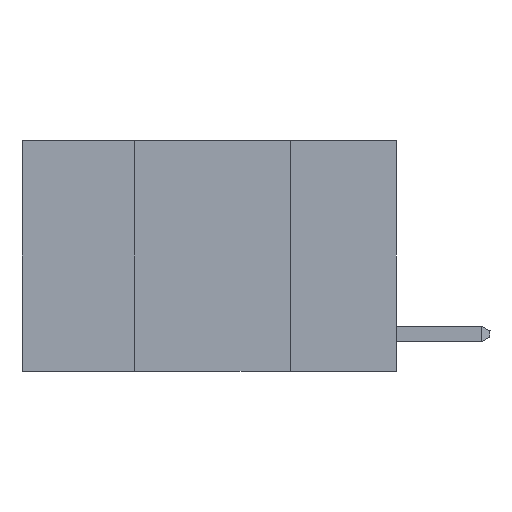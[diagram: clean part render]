
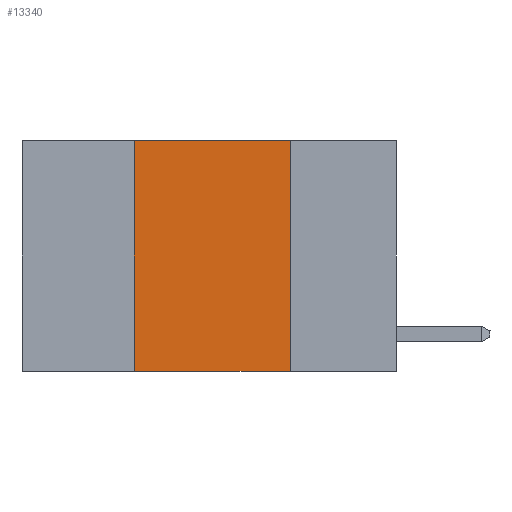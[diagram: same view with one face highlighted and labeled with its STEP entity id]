
A CAD part, left-side view. The second image highlights one B-rep face of the part: STEP entity #13340.
In plain terms, the highlighted planar face has unit normal (-1, 0, 0).
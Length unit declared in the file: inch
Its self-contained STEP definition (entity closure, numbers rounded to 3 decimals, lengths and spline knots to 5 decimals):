
#36 = DIRECTION ( 'NONE',  ( 0., -1., 0. ) ) ;
#970 = EDGE_CURVE ( 'NONE', #9178, #13717, #9839, .T. ) ;
#1294 = VERTEX_POINT ( 'NONE', #14697 ) ;
#2353 = ORIENTED_EDGE ( 'NONE', *, *, #5533, .F. ) ;
#3614 = VECTOR ( 'NONE', #36, 39.37008 ) ;
#3980 = VECTOR ( 'NONE', #14433, 39.37008 ) ;
#4846 = AXIS2_PLACEMENT_3D ( 'NONE', #16590, #19564, #6936 ) ;
#5307 = PLANE ( 'NONE',  #4846 ) ;
#5533 = EDGE_CURVE ( 'NONE', #12806, #9178, #7271, .T. ) ;
#6019 = ORIENTED_EDGE ( 'NONE', *, *, #19326, .F. ) ;
#6936 = DIRECTION ( 'NONE',  ( 0., 0., -1. ) ) ;
#7180 = CARTESIAN_POINT ( 'NONE',  ( 0., 0.6, 0. ) ) ;
#7271 = LINE ( 'NONE', #19435, #3980 ) ;
#8735 = FACE_OUTER_BOUND ( 'NONE', #16406, .T. ) ;
#8837 = DIRECTION ( 'NONE',  ( 0., -1., 0. ) ) ;
#9178 = VERTEX_POINT ( 'NONE', #11370 ) ;
#9364 = CARTESIAN_POINT ( 'NONE',  ( 0., 0.6, -0.37 ) ) ;
#9707 = VECTOR ( 'NONE', #18661, 39.37008 ) ;
#9781 = CARTESIAN_POINT ( 'NONE',  ( 0., 0.17, 0. ) ) ;
#9839 = LINE ( 'NONE', #7180, #17829 ) ;
#9998 = CARTESIAN_POINT ( 'NONE',  ( 0., 0.17, 0. ) ) ;
#11370 = CARTESIAN_POINT ( 'NONE',  ( 0., 0.42, 0. ) ) ;
#12806 = VERTEX_POINT ( 'NONE', #15641 ) ;
#13340 = ADVANCED_FACE ( 'NONE', ( #8735 ), #5307, .F. ) ;
#13495 = LINE ( 'NONE', #9364, #3614 ) ;
#13717 = VERTEX_POINT ( 'NONE', #9998 ) ;
#14175 = ORIENTED_EDGE ( 'NONE', *, *, #18818, .T. ) ;
#14240 = LINE ( 'NONE', #9781, #9707 ) ;
#14433 = DIRECTION ( 'NONE',  ( 0., 0., 1. ) ) ;
#14697 = CARTESIAN_POINT ( 'NONE',  ( 0., 0.17, -0.37 ) ) ;
#15641 = CARTESIAN_POINT ( 'NONE',  ( 0., 0.42, -0.37 ) ) ;
#15824 = ORIENTED_EDGE ( 'NONE', *, *, #970, .F. ) ;
#16406 = EDGE_LOOP ( 'NONE', ( #6019, #15824, #2353, #14175 ) ) ;
#16590 = CARTESIAN_POINT ( 'NONE',  ( 0., 0.6, 0. ) ) ;
#17829 = VECTOR ( 'NONE', #8837, 39.37008 ) ;
#18661 = DIRECTION ( 'NONE',  ( 0., 0., -1. ) ) ;
#18818 = EDGE_CURVE ( 'NONE', #12806, #1294, #13495, .T. ) ;
#19326 = EDGE_CURVE ( 'NONE', #13717, #1294, #14240, .T. ) ;
#19435 = CARTESIAN_POINT ( 'NONE',  ( 0., 0.42, 0. ) ) ;
#19564 = DIRECTION ( 'NONE',  ( 1., 0., 0. ) ) ;
